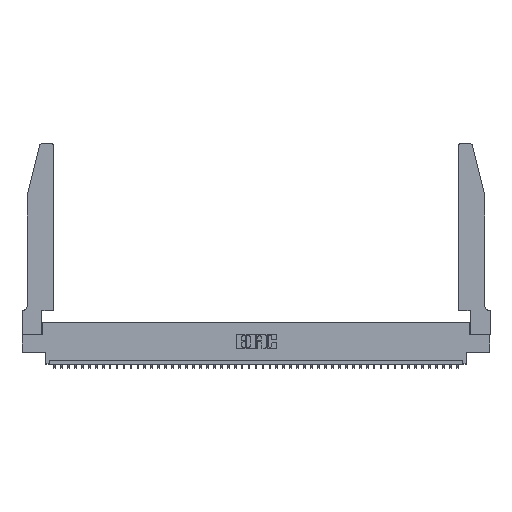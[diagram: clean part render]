
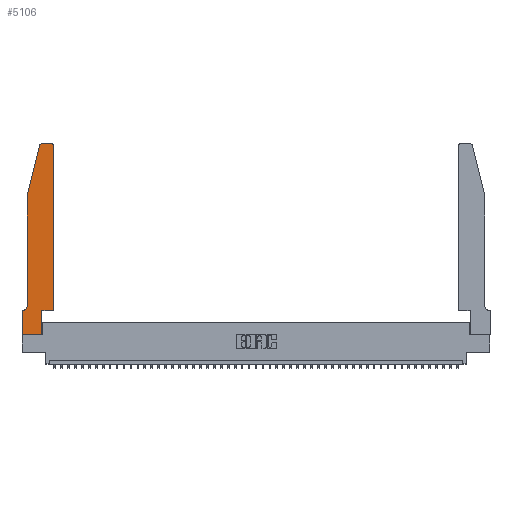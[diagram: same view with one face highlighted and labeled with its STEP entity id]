
A CAD part, top view. The second image highlights one B-rep face of the part: STEP entity #5106.
In plain terms, the highlighted planar face has unit normal (0, 0, 1).
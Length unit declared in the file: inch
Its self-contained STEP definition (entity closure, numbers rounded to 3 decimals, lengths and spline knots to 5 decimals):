
#31 = LINE ( 'NONE', #19283, #25677 ) ;
#242 = CARTESIAN_POINT ( 'NONE',  ( 0.2865, 0.35, 0.37 ) ) ;
#1175 = EDGE_CURVE ( 'NONE', #24565, #30249, #31, .T. ) ;
#1356 = DIRECTION ( 'NONE',  ( 1., 0., 0. ) ) ;
#1601 = DIRECTION ( 'NONE',  ( 0., 0., 1. ) ) ;
#1730 = DIRECTION ( 'NONE',  ( -1., 0., 0. ) ) ;
#2354 = EDGE_CURVE ( 'NONE', #40568, #18496, #13720, .T. ) ;
#2904 = DIRECTION ( 'NONE',  ( 0., -1., 0. ) ) ;
#3023 = ORIENTED_EDGE ( 'NONE', *, *, #30651, .T. ) ;
#3414 = CARTESIAN_POINT ( 'NONE',  ( 0., 0., 0.37 ) ) ;
#3604 = EDGE_CURVE ( 'NONE', #30249, #26224, #30056, .T. ) ;
#4137 = VECTOR ( 'NONE', #16802, 39.37008 ) ;
#4255 = CARTESIAN_POINT ( 'NONE',  ( 0.0755, 0.42, 0.37 ) ) ;
#4641 = VERTEX_POINT ( 'NONE', #42446 ) ;
#4682 = CARTESIAN_POINT ( 'NONE',  ( 0.25487, 2.72718, 0.37 ) ) ;
#4736 = LINE ( 'NONE', #33928, #46200 ) ;
#5106 = ADVANCED_FACE ( 'NONE', ( #34350 ), #12198, .T. ) ;
#5365 = ORIENTED_EDGE ( 'NONE', *, *, #19026, .T. ) ;
#5460 = VECTOR ( 'NONE', #11992, 39.37008 ) ;
#5878 = LINE ( 'NONE', #11822, #43330 ) ;
#5880 = VECTOR ( 'NONE', #10878, 39.37008 ) ;
#6578 = EDGE_CURVE ( 'NONE', #18496, #24565, #31988, .T. ) ;
#7825 = VERTEX_POINT ( 'NONE', #42279 ) ;
#7910 = VERTEX_POINT ( 'NONE', #46539 ) ;
#8300 = CARTESIAN_POINT ( 'NONE',  ( 0.4505, 2.72, 0.37 ) ) ;
#8324 = DIRECTION ( 'NONE',  ( -1., 0., 0. ) ) ;
#8631 = DIRECTION ( 'NONE',  ( 0., 0., -1. ) ) ;
#9949 = ORIENTED_EDGE ( 'NONE', *, *, #1175, .T. ) ;
#10328 = DIRECTION ( 'NONE',  ( 0., 0., 1. ) ) ;
#10710 = ORIENTED_EDGE ( 'NONE', *, *, #6578, .T. ) ;
#10878 = DIRECTION ( 'NONE',  ( -0.239, -0.971, 0. ) ) ;
#11538 = ORIENTED_EDGE ( 'NONE', *, *, #25363, .T. ) ;
#11822 = CARTESIAN_POINT ( 'NONE',  ( 0.2605, 2.75, 0.37 ) ) ;
#11992 = DIRECTION ( 'NONE',  ( 1., 0., 0. ) ) ;
#12198 = PLANE ( 'NONE',  #32517 ) ;
#13720 = LINE ( 'NONE', #19774, #42618 ) ;
#13845 = LINE ( 'NONE', #15027, #5880 ) ;
#14325 = ORIENTED_EDGE ( 'NONE', *, *, #3604, .T. ) ;
#14464 = VERTEX_POINT ( 'NONE', #8300 ) ;
#14993 = VERTEX_POINT ( 'NONE', #19953 ) ;
#15027 = CARTESIAN_POINT ( 'NONE',  ( 0.0755, 2., 0.37 ) ) ;
#15851 = CARTESIAN_POINT ( 'NONE',  ( 0.4205, 2.72, 0.37 ) ) ;
#16802 = DIRECTION ( 'NONE',  ( 0., 1., 0. ) ) ;
#17493 = ORIENTED_EDGE ( 'NONE', *, *, #42063, .T. ) ;
#18496 = VERTEX_POINT ( 'NONE', #4255 ) ;
#19026 = EDGE_CURVE ( 'NONE', #7910, #4641, #5878, .T. ) ;
#19283 = CARTESIAN_POINT ( 'NONE',  ( 0.0755, 0.35, 0.37 ) ) ;
#19328 = ORIENTED_EDGE ( 'NONE', *, *, #24196, .T. ) ;
#19470 = DIRECTION ( 'NONE',  ( 1., 0., 0. ) ) ;
#19626 = CARTESIAN_POINT ( 'NONE',  ( 0., 0.35, 0.37 ) ) ;
#19774 = CARTESIAN_POINT ( 'NONE',  ( 0.0755, 2., 0.37 ) ) ;
#19953 = CARTESIAN_POINT ( 'NONE',  ( 0.4505, 0.35, 0.37 ) ) ;
#20104 = AXIS2_PLACEMENT_3D ( 'NONE', #32661, #36268, #29044 ) ;
#22001 = CIRCLE ( 'NONE', #20104, 0.03 ) ;
#23554 = LINE ( 'NONE', #35137, #4137 ) ;
#24196 = EDGE_CURVE ( 'NONE', #14464, #7910, #40498, .T. ) ;
#24279 = CARTESIAN_POINT ( 'NONE',  ( 0.0055, 0.35, 0.37 ) ) ;
#24565 = VERTEX_POINT ( 'NONE', #24279 ) ;
#24777 = ORIENTED_EDGE ( 'NONE', *, *, #25443, .T. ) ;
#25154 = EDGE_CURVE ( 'NONE', #26224, #7825, #4736, .T. ) ;
#25242 = CARTESIAN_POINT ( 'NONE',  ( 0., 0.35, 0.37 ) ) ;
#25338 = CARTESIAN_POINT ( 'NONE',  ( 0.4505, 0.35, 0.37 ) ) ;
#25363 = EDGE_CURVE ( 'NONE', #14993, #14464, #23554, .T. ) ;
#25396 = DIRECTION ( 'NONE',  ( 1., 0., 0. ) ) ;
#25443 = EDGE_CURVE ( 'NONE', #42801, #40568, #13845, .T. ) ;
#25554 = EDGE_LOOP ( 'NONE', ( #5365, #3023, #24777, #33911, #10710, #9949, #14325, #30258, #17493, #35242, #11538, #19328 ) ) ;
#25677 = VECTOR ( 'NONE', #8324, 39.37008 ) ;
#26216 = DIRECTION ( 'NONE',  ( 0., 1., 0. ) ) ;
#26224 = VERTEX_POINT ( 'NONE', #3414 ) ;
#27444 = AXIS2_PLACEMENT_3D ( 'NONE', #30387, #8631, #1730 ) ;
#29044 = DIRECTION ( 'NONE',  ( 1., 0., 0. ) ) ;
#30056 = LINE ( 'NONE', #38915, #30605 ) ;
#30249 = VERTEX_POINT ( 'NONE', #19626 ) ;
#30258 = ORIENTED_EDGE ( 'NONE', *, *, #25154, .T. ) ;
#30387 = CARTESIAN_POINT ( 'NONE',  ( 0.0055, 0.42, 0.37 ) ) ;
#30605 = VECTOR ( 'NONE', #2904, 39.37008 ) ;
#30651 = EDGE_CURVE ( 'NONE', #4641, #42801, #22001, .T. ) ;
#30736 = VECTOR ( 'NONE', #26216, 39.37008 ) ;
#31988 = CIRCLE ( 'NONE', #27444, 0.07 ) ;
#32517 = AXIS2_PLACEMENT_3D ( 'NONE', #25242, #10328, #25396 ) ;
#32661 = CARTESIAN_POINT ( 'NONE',  ( 0.284, 2.72, 0.37 ) ) ;
#33911 = ORIENTED_EDGE ( 'NONE', *, *, #2354, .T. ) ;
#33928 = CARTESIAN_POINT ( 'NONE',  ( 0., 0., 0.37 ) ) ;
#34199 = VERTEX_POINT ( 'NONE', #46196 ) ;
#34323 = DIRECTION ( 'NONE',  ( 0., -1., 0. ) ) ;
#34334 = DIRECTION ( 'NONE',  ( -1., 0., 0. ) ) ;
#34350 = FACE_OUTER_BOUND ( 'NONE', #25554, .T. ) ;
#35137 = CARTESIAN_POINT ( 'NONE',  ( 0.4505, 0.35, 0.37 ) ) ;
#35235 = LINE ( 'NONE', #242, #30736 ) ;
#35242 = ORIENTED_EDGE ( 'NONE', *, *, #43256, .T. ) ;
#36268 = DIRECTION ( 'NONE',  ( 0., 0., 1. ) ) ;
#38915 = CARTESIAN_POINT ( 'NONE',  ( 0., 0., 0.37 ) ) ;
#39931 = CARTESIAN_POINT ( 'NONE',  ( 0.0755, 2., 0.37 ) ) ;
#39986 = AXIS2_PLACEMENT_3D ( 'NONE', #15851, #1601, #19470 ) ;
#40498 = CIRCLE ( 'NONE', #39986, 0.03 ) ;
#40568 = VERTEX_POINT ( 'NONE', #39931 ) ;
#41804 = LINE ( 'NONE', #25338, #5460 ) ;
#42063 = EDGE_CURVE ( 'NONE', #7825, #34199, #35235, .T. ) ;
#42279 = CARTESIAN_POINT ( 'NONE',  ( 0.2865, 0., 0.37 ) ) ;
#42446 = CARTESIAN_POINT ( 'NONE',  ( 0.284, 2.75, 0.37 ) ) ;
#42618 = VECTOR ( 'NONE', #34323, 39.37008 ) ;
#42801 = VERTEX_POINT ( 'NONE', #4682 ) ;
#43256 = EDGE_CURVE ( 'NONE', #34199, #14993, #41804, .T. ) ;
#43330 = VECTOR ( 'NONE', #34334, 39.37008 ) ;
#46196 = CARTESIAN_POINT ( 'NONE',  ( 0.2865, 0.35, 0.37 ) ) ;
#46200 = VECTOR ( 'NONE', #1356, 39.37008 ) ;
#46539 = CARTESIAN_POINT ( 'NONE',  ( 0.4205, 2.75, 0.37 ) ) ;
